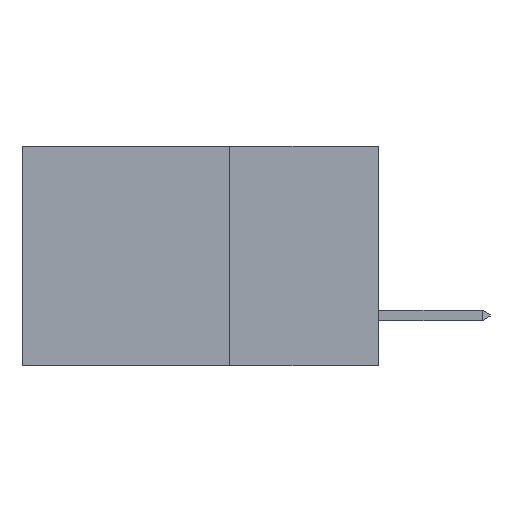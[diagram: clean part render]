
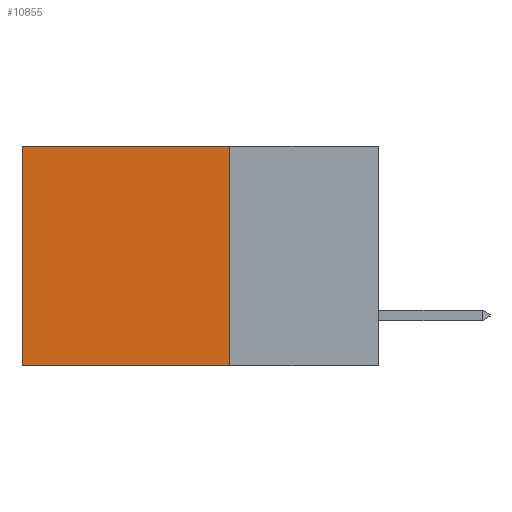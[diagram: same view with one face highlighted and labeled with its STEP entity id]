
A CAD part, left-side view. The second image highlights one B-rep face of the part: STEP entity #10855.
In plain terms, the highlighted planar face has unit normal (-1, 0, 0).
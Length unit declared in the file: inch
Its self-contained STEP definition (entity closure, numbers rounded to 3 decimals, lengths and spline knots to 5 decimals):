
#1874 = ORIENTED_EDGE ( 'NONE', *, *, #19229, .T. ) ;
#3074 = PLANE ( 'NONE',  #4040 ) ;
#3951 = DIRECTION ( 'NONE',  ( 0., 0., -1. ) ) ;
#4040 = AXIS2_PLACEMENT_3D ( 'NONE', #14401, #15949, #6424 ) ;
#4043 = CARTESIAN_POINT ( 'NONE',  ( 0.298, 0.25, -0.37 ) ) ;
#5432 = DIRECTION ( 'NONE',  ( 0., 0., -1. ) ) ;
#5685 = CARTESIAN_POINT ( 'NONE',  ( 0.298, 0.25, 0. ) ) ;
#6243 = EDGE_CURVE ( 'NONE', #12914, #16180, #18469, .T. ) ;
#6424 = DIRECTION ( 'NONE',  ( 0., 0., -1. ) ) ;
#7190 = LINE ( 'NONE', #13488, #14651 ) ;
#7591 = EDGE_CURVE ( 'NONE', #9647, #12914, #13721, .T. ) ;
#7854 = FACE_OUTER_BOUND ( 'NONE', #12175, .T. ) ;
#7865 = VECTOR ( 'NONE', #20654, 39.37008 ) ;
#8581 = CARTESIAN_POINT ( 'NONE',  ( 0.298, 0.6, 0. ) ) ;
#8982 = VECTOR ( 'NONE', #3951, 39.37008 ) ;
#9568 = CARTESIAN_POINT ( 'NONE',  ( 0.298, 0.25, 0. ) ) ;
#9647 = VERTEX_POINT ( 'NONE', #9791 ) ;
#9791 = CARTESIAN_POINT ( 'NONE',  ( 0.298, 0.25, 0. ) ) ;
#10142 = DIRECTION ( 'NONE',  ( 0., 1., 0. ) ) ;
#10855 = ADVANCED_FACE ( 'NONE', ( #7854 ), #3074, .F. ) ;
#12175 = EDGE_LOOP ( 'NONE', ( #1874, #19322, #13250, #19148 ) ) ;
#12914 = VERTEX_POINT ( 'NONE', #4043 ) ;
#13250 = ORIENTED_EDGE ( 'NONE', *, *, #7591, .F. ) ;
#13488 = CARTESIAN_POINT ( 'NONE',  ( 0.298, 0.6, 0. ) ) ;
#13721 = LINE ( 'NONE', #5685, #8982 ) ;
#13782 = VECTOR ( 'NONE', #10142, 39.37008 ) ;
#14401 = CARTESIAN_POINT ( 'NONE',  ( 0.298, 0.25, 0. ) ) ;
#14651 = VECTOR ( 'NONE', #5432, 39.37008 ) ;
#15173 = VERTEX_POINT ( 'NONE', #8581 ) ;
#15570 = EDGE_CURVE ( 'NONE', #9647, #15173, #16224, .T. ) ;
#15949 = DIRECTION ( 'NONE',  ( 1., 0., 0. ) ) ;
#16180 = VERTEX_POINT ( 'NONE', #18953 ) ;
#16224 = LINE ( 'NONE', #9568, #7865 ) ;
#17207 = CARTESIAN_POINT ( 'NONE',  ( 0.298, 0.25, -0.37 ) ) ;
#18469 = LINE ( 'NONE', #17207, #13782 ) ;
#18953 = CARTESIAN_POINT ( 'NONE',  ( 0.298, 0.6, -0.37 ) ) ;
#19148 = ORIENTED_EDGE ( 'NONE', *, *, #15570, .T. ) ;
#19229 = EDGE_CURVE ( 'NONE', #15173, #16180, #7190, .T. ) ;
#19322 = ORIENTED_EDGE ( 'NONE', *, *, #6243, .F. ) ;
#20654 = DIRECTION ( 'NONE',  ( 0., 1., 0. ) ) ;
